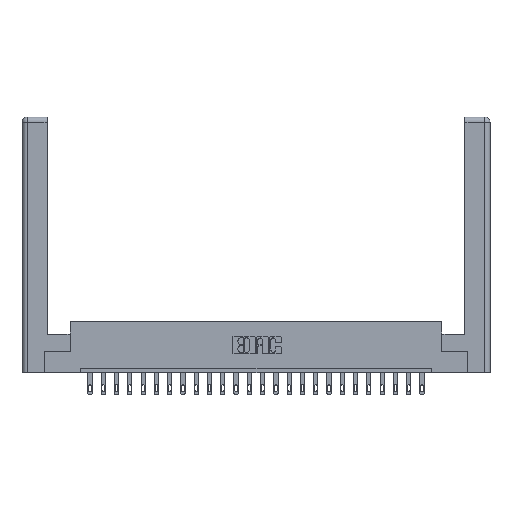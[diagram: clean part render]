
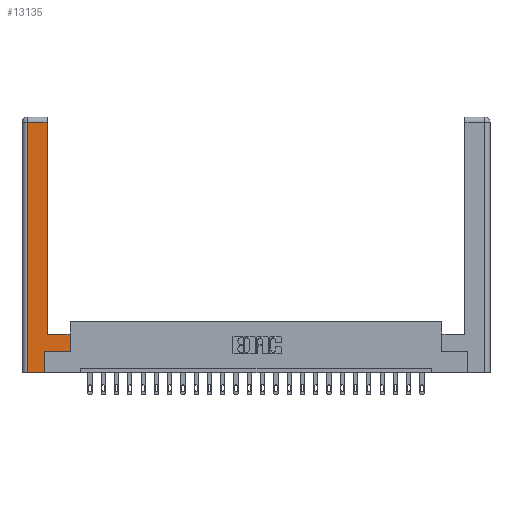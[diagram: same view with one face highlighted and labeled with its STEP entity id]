
A CAD part, top view. The second image highlights one B-rep face of the part: STEP entity #13135.
In plain terms, the highlighted planar face has unit normal (0, 0, 1).
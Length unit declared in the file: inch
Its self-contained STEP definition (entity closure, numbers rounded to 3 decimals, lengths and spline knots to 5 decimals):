
#168 = LINE ( 'NONE', #15317, #14389 ) ;
#300 = VERTEX_POINT ( 'NONE', #21255 ) ;
#730 = ORIENTED_EDGE ( 'NONE', *, *, #5423, .T. ) ;
#798 = CARTESIAN_POINT ( 'NONE',  ( 0.565, 0.245, 0. ) ) ;
#856 = LINE ( 'NONE', #23130, #20534 ) ;
#1077 = EDGE_LOOP ( 'NONE', ( #5289, #22688, #12181, #730, #15965, #5655, #1865, #21966 ) ) ;
#1865 = ORIENTED_EDGE ( 'NONE', *, *, #18263, .T. ) ;
#1994 = LINE ( 'NONE', #21973, #21095 ) ;
#2130 = FACE_OUTER_BOUND ( 'NONE', #1077, .T. ) ;
#4220 = EDGE_CURVE ( 'NONE', #21795, #11532, #20155, .T. ) ;
#4556 = CARTESIAN_POINT ( 'NONE',  ( 0.0615, 0., 0. ) ) ;
#4587 = DIRECTION ( 'NONE',  ( 0., -1., 0. ) ) ;
#5289 = ORIENTED_EDGE ( 'NONE', *, *, #22426, .T. ) ;
#5423 = EDGE_CURVE ( 'NONE', #16181, #300, #12273, .T. ) ;
#5655 = ORIENTED_EDGE ( 'NONE', *, *, #4220, .T. ) ;
#6226 = VERTEX_POINT ( 'NONE', #16093 ) ;
#6410 = CARTESIAN_POINT ( 'NONE',  ( 0.265, 0., 0. ) ) ;
#7223 = LINE ( 'NONE', #10973, #20221 ) ;
#7708 = DIRECTION ( 'NONE',  ( -1., 0., 0. ) ) ;
#7814 = CARTESIAN_POINT ( 'NONE',  ( 0.295, 0.45, 0. ) ) ;
#8301 = DIRECTION ( 'NONE',  ( 1., 0., 0. ) ) ;
#10339 = CARTESIAN_POINT ( 'NONE',  ( 0.295, 3., 0. ) ) ;
#10413 = LINE ( 'NONE', #13912, #22544 ) ;
#10973 = CARTESIAN_POINT ( 'NONE',  ( 0.295, 0.45, 0. ) ) ;
#11337 = CARTESIAN_POINT ( 'NONE',  ( 0., 0., 0. ) ) ;
#11532 = VERTEX_POINT ( 'NONE', #17925 ) ;
#11813 = DIRECTION ( 'NONE',  ( -1., 0., 0. ) ) ;
#11956 = DIRECTION ( 'NONE',  ( 0., 1., 0. ) ) ;
#12181 = ORIENTED_EDGE ( 'NONE', *, *, #18098, .T. ) ;
#12273 = LINE ( 'NONE', #6410, #18600 ) ;
#12744 = CARTESIAN_POINT ( 'NONE',  ( 0.295, 2.94, 0. ) ) ;
#12803 = EDGE_CURVE ( 'NONE', #300, #21795, #168, .T. ) ;
#13135 = ADVANCED_FACE ( 'NONE', ( #2130 ), #18764, .F. ) ;
#13742 = CARTESIAN_POINT ( 'NONE',  ( 0.565, 0.45, 0. ) ) ;
#13912 = CARTESIAN_POINT ( 'NONE',  ( 0.0615, 0., 0. ) ) ;
#14389 = VECTOR ( 'NONE', #15858, 39.37008 ) ;
#14642 = VERTEX_POINT ( 'NONE', #12744 ) ;
#15317 = CARTESIAN_POINT ( 'NONE',  ( 0.265, 0.245, 0. ) ) ;
#15737 = EDGE_CURVE ( 'NONE', #14642, #6226, #856, .T. ) ;
#15858 = DIRECTION ( 'NONE',  ( 0., 1., 0. ) ) ;
#15965 = ORIENTED_EDGE ( 'NONE', *, *, #12803, .T. ) ;
#16093 = CARTESIAN_POINT ( 'NONE',  ( 0.0615, 2.94, 0. ) ) ;
#16135 = VECTOR ( 'NONE', #11956, 39.37008 ) ;
#16181 = VERTEX_POINT ( 'NONE', #4556 ) ;
#16461 = DIRECTION ( 'NONE',  ( -1., 0., 0. ) ) ;
#17052 = DIRECTION ( 'NONE',  ( 0., 0., -1. ) ) ;
#17094 = AXIS2_PLACEMENT_3D ( 'NONE', #11337, #17052, #7708 ) ;
#17869 = CARTESIAN_POINT ( 'NONE',  ( 0.265, 0.245, 0. ) ) ;
#17925 = CARTESIAN_POINT ( 'NONE',  ( 0.565, 0.245, 0. ) ) ;
#18098 = EDGE_CURVE ( 'NONE', #6226, #16181, #10413, .T. ) ;
#18154 = LINE ( 'NONE', #10339, #16135 ) ;
#18263 = EDGE_CURVE ( 'NONE', #11532, #19671, #1994, .T. ) ;
#18435 = EDGE_CURVE ( 'NONE', #19671, #22180, #7223, .T. ) ;
#18600 = VECTOR ( 'NONE', #8301, 39.37008 ) ;
#18764 = PLANE ( 'NONE',  #17094 ) ;
#19396 = DIRECTION ( 'NONE',  ( 1., 0., 0. ) ) ;
#19671 = VERTEX_POINT ( 'NONE', #13742 ) ;
#20155 = LINE ( 'NONE', #798, #23619 ) ;
#20221 = VECTOR ( 'NONE', #16461, 39.37008 ) ;
#20534 = VECTOR ( 'NONE', #11813, 39.37008 ) ;
#21095 = VECTOR ( 'NONE', #21664, 39.37008 ) ;
#21255 = CARTESIAN_POINT ( 'NONE',  ( 0.265, 0., 0. ) ) ;
#21664 = DIRECTION ( 'NONE',  ( 0., 1., 0. ) ) ;
#21795 = VERTEX_POINT ( 'NONE', #17869 ) ;
#21966 = ORIENTED_EDGE ( 'NONE', *, *, #18435, .T. ) ;
#21973 = CARTESIAN_POINT ( 'NONE',  ( 0.565, 0.45, 0. ) ) ;
#22180 = VERTEX_POINT ( 'NONE', #7814 ) ;
#22426 = EDGE_CURVE ( 'NONE', #22180, #14642, #18154, .T. ) ;
#22544 = VECTOR ( 'NONE', #4587, 39.37008 ) ;
#22688 = ORIENTED_EDGE ( 'NONE', *, *, #15737, .T. ) ;
#23130 = CARTESIAN_POINT ( 'NONE',  ( 0.0615, 2.94, 0. ) ) ;
#23619 = VECTOR ( 'NONE', #19396, 39.37008 ) ;
